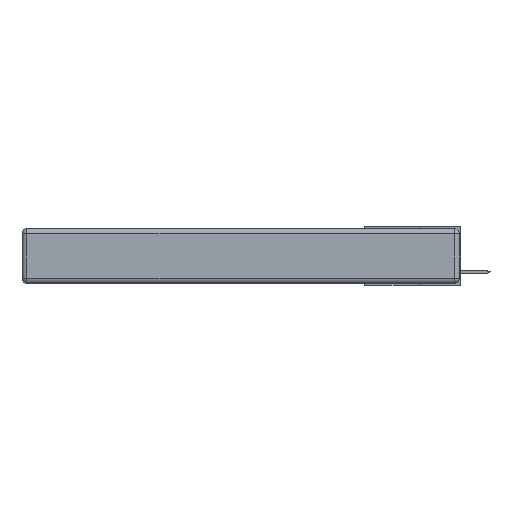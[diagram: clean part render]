
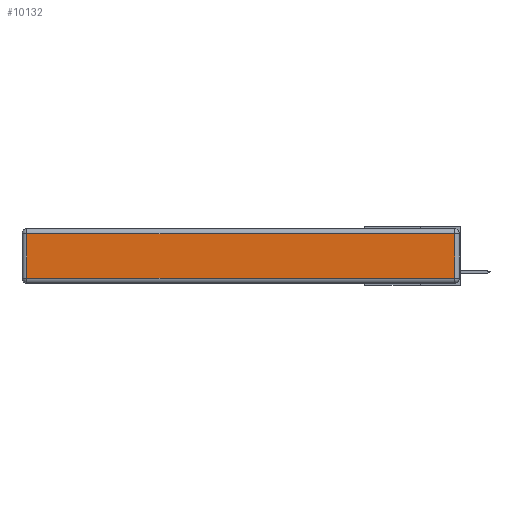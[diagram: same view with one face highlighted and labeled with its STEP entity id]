
A CAD part, left-side view. The second image highlights one B-rep face of the part: STEP entity #10132.
In plain terms, the highlighted planar face has unit normal (-1, 0, 0).
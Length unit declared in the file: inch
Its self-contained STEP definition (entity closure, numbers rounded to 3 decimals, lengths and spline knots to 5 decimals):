
#98 = ORIENTED_EDGE ( 'NONE', *, *, #11233, .T. ) ;
#513 = DIRECTION ( 'NONE',  ( 0., -1., 0. ) ) ;
#879 = VECTOR ( 'NONE', #12109, 39.37008 ) ;
#966 = AXIS2_PLACEMENT_3D ( 'NONE', #3423, #5402, #12856 ) ;
#1219 = LINE ( 'NONE', #12932, #10059 ) ;
#2106 = ORIENTED_EDGE ( 'NONE', *, *, #5490, .T. ) ;
#2565 = CARTESIAN_POINT ( 'NONE',  ( 0., 0., -0.313 ) ) ;
#3017 = EDGE_LOOP ( 'NONE', ( #4244, #12356, #98, #2106 ) ) ;
#3423 = CARTESIAN_POINT ( 'NONE',  ( 0., 0., -0.343 ) ) ;
#3781 = CARTESIAN_POINT ( 'NONE',  ( 0., 0.03, -0.343 ) ) ;
#3944 = VERTEX_POINT ( 'NONE', #4937 ) ;
#4244 = ORIENTED_EDGE ( 'NONE', *, *, #6373, .T. ) ;
#4276 = CARTESIAN_POINT ( 'NONE',  ( 0., 2.72, -0.313 ) ) ;
#4835 = FACE_OUTER_BOUND ( 'NONE', #3017, .T. ) ;
#4855 = VECTOR ( 'NONE', #513, 39.37008 ) ;
#4937 = CARTESIAN_POINT ( 'NONE',  ( 0., 0.03, -0.313 ) ) ;
#5091 = EDGE_CURVE ( 'NONE', #3944, #5548, #5933, .T. ) ;
#5147 = VECTOR ( 'NONE', #10392, 39.37008 ) ;
#5402 = DIRECTION ( 'NONE',  ( -1., 0., 0. ) ) ;
#5490 = EDGE_CURVE ( 'NONE', #8294, #5551, #1219, .T. ) ;
#5548 = VERTEX_POINT ( 'NONE', #7643 ) ;
#5551 = VERTEX_POINT ( 'NONE', #4276 ) ;
#5933 = LINE ( 'NONE', #3781, #879 ) ;
#6373 = EDGE_CURVE ( 'NONE', #5551, #3944, #7054, .T. ) ;
#7054 = LINE ( 'NONE', #2565, #4855 ) ;
#7643 = CARTESIAN_POINT ( 'NONE',  ( 0., 0.03, -0.03 ) ) ;
#8294 = VERTEX_POINT ( 'NONE', #9471 ) ;
#8672 = DIRECTION ( 'NONE',  ( 0., 0., -1. ) ) ;
#9471 = CARTESIAN_POINT ( 'NONE',  ( 0., 2.72, -0.03 ) ) ;
#9723 = PLANE ( 'NONE',  #966 ) ;
#10059 = VECTOR ( 'NONE', #8672, 39.37008 ) ;
#10132 = ADVANCED_FACE ( 'NONE', ( #4835 ), #9723, .T. ) ;
#10392 = DIRECTION ( 'NONE',  ( 0., 1., 0. ) ) ;
#11171 = LINE ( 'NONE', #11632, #5147 ) ;
#11233 = EDGE_CURVE ( 'NONE', #5548, #8294, #11171, .T. ) ;
#11632 = CARTESIAN_POINT ( 'NONE',  ( 0., 2.75, -0.03 ) ) ;
#12109 = DIRECTION ( 'NONE',  ( 0., 0., 1. ) ) ;
#12356 = ORIENTED_EDGE ( 'NONE', *, *, #5091, .T. ) ;
#12856 = DIRECTION ( 'NONE',  ( 0., 0., 1. ) ) ;
#12932 = CARTESIAN_POINT ( 'NONE',  ( 0., 2.72, -0.343 ) ) ;
